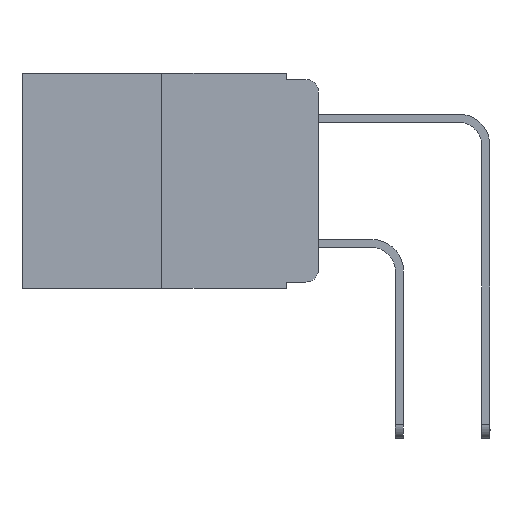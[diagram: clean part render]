
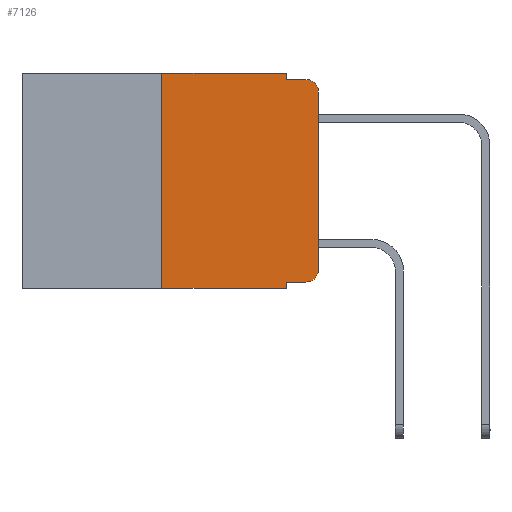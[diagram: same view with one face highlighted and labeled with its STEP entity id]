
A CAD part, left-side view. The second image highlights one B-rep face of the part: STEP entity #7126.
In plain terms, the highlighted planar face has unit normal (-1, 0, 0).
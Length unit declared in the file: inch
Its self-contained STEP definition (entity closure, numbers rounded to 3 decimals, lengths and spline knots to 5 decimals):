
#62 = ORIENTED_EDGE ( 'NONE', *, *, #11302, .T. ) ;
#249 = CARTESIAN_POINT ( 'NONE',  ( 0., 0.051, -0.01 ) ) ;
#327 = PLANE ( 'NONE',  #916 ) ;
#438 = AXIS2_PLACEMENT_3D ( 'NONE', #8226, #11312, #13132 ) ;
#916 = AXIS2_PLACEMENT_3D ( 'NONE', #1693, #9468, #11037 ) ;
#928 = DIRECTION ( 'NONE',  ( 0., 0., -1. ) ) ;
#1140 = LINE ( 'NONE', #249, #10842 ) ;
#1475 = CIRCLE ( 'NONE', #12382, 0.02 ) ;
#1693 = CARTESIAN_POINT ( 'NONE',  ( 0., 0.473, 0. ) ) ;
#1869 = EDGE_CURVE ( 'NONE', #2142, #2670, #3635, .T. ) ;
#2142 = VERTEX_POINT ( 'NONE', #12959 ) ;
#2294 = ORIENTED_EDGE ( 'NONE', *, *, #1869, .F. ) ;
#2642 = ORIENTED_EDGE ( 'NONE', *, *, #11221, .T. ) ;
#2658 = ORIENTED_EDGE ( 'NONE', *, *, #2874, .F. ) ;
#2670 = VERTEX_POINT ( 'NONE', #5640 ) ;
#2736 = VERTEX_POINT ( 'NONE', #5255 ) ;
#2874 = EDGE_CURVE ( 'NONE', #3925, #13097, #16921, .T. ) ;
#3635 = LINE ( 'NONE', #16708, #6300 ) ;
#3925 = VERTEX_POINT ( 'NONE', #10265 ) ;
#3939 = ORIENTED_EDGE ( 'NONE', *, *, #9696, .T. ) ;
#4692 = VERTEX_POINT ( 'NONE', #11938 ) ;
#4830 = CARTESIAN_POINT ( 'NONE',  ( 0., 0.25, -0.343 ) ) ;
#5009 = CARTESIAN_POINT ( 'NONE',  ( 0., 0.25, 0. ) ) ;
#5255 = CARTESIAN_POINT ( 'NONE',  ( 0., 0.02, -0.333 ) ) ;
#5284 = CARTESIAN_POINT ( 'NONE',  ( 0., 0.473, -0.343 ) ) ;
#5640 = CARTESIAN_POINT ( 'NONE',  ( 0., 0.051, -0.01 ) ) ;
#5737 = DIRECTION ( 'NONE',  ( 0., 0., -1. ) ) ;
#5816 = EDGE_CURVE ( 'NONE', #4692, #2142, #19254, .T. ) ;
#5990 = VECTOR ( 'NONE', #17746, 39.37008 ) ;
#6300 = VECTOR ( 'NONE', #19614, 39.37008 ) ;
#6592 = ORIENTED_EDGE ( 'NONE', *, *, #7976, .F. ) ;
#7126 = ADVANCED_FACE ( 'NONE', ( #15582 ), #327, .F. ) ;
#7976 = EDGE_CURVE ( 'NONE', #19413, #4692, #19197, .T. ) ;
#8202 = CARTESIAN_POINT ( 'NONE',  ( 0., 0., -0.313 ) ) ;
#8226 = CARTESIAN_POINT ( 'NONE',  ( 0., 0.02, -0.03 ) ) ;
#8430 = DIRECTION ( 'NONE',  ( -1., 0., 0. ) ) ;
#8497 = ORIENTED_EDGE ( 'NONE', *, *, #8825, .T. ) ;
#8541 = CARTESIAN_POINT ( 'NONE',  ( 0., 0.051, -0.333 ) ) ;
#8825 = EDGE_CURVE ( 'NONE', #2736, #11084, #1475, .T. ) ;
#9330 = EDGE_LOOP ( 'NONE', ( #16702, #3939, #11700, #2294, #16888, #6592, #62, #2658, #2642, #8497 ) ) ;
#9412 = VECTOR ( 'NONE', #5737, 39.37008 ) ;
#9468 = DIRECTION ( 'NONE',  ( 1., 0., 0. ) ) ;
#9590 = LINE ( 'NONE', #14490, #16376 ) ;
#9653 = DIRECTION ( 'NONE',  ( 0., -1., 0. ) ) ;
#9696 = EDGE_CURVE ( 'NONE', #13938, #11615, #12123, .T. ) ;
#9826 = DIRECTION ( 'NONE',  ( 0., -1., 0. ) ) ;
#10048 = VECTOR ( 'NONE', #10253, 39.37008 ) ;
#10253 = DIRECTION ( 'NONE',  ( 0., -1., 0. ) ) ;
#10265 = CARTESIAN_POINT ( 'NONE',  ( 0., 0.051, -0.333 ) ) ;
#10842 = VECTOR ( 'NONE', #9653, 39.37008 ) ;
#11037 = DIRECTION ( 'NONE',  ( 0., 0., -1. ) ) ;
#11084 = VERTEX_POINT ( 'NONE', #8202 ) ;
#11221 = EDGE_CURVE ( 'NONE', #3925, #2736, #18585, .T. ) ;
#11302 = EDGE_CURVE ( 'NONE', #19413, #13097, #16900, .T. ) ;
#11312 = DIRECTION ( 'NONE',  ( -1., 0., 0. ) ) ;
#11615 = VERTEX_POINT ( 'NONE', #16879 ) ;
#11700 = ORIENTED_EDGE ( 'NONE', *, *, #15990, .F. ) ;
#11822 = EDGE_CURVE ( 'NONE', #11084, #13938, #9590, .T. ) ;
#11938 = CARTESIAN_POINT ( 'NONE',  ( 0., 0.25, 0. ) ) ;
#12123 = CIRCLE ( 'NONE', #438, 0.02 ) ;
#12187 = CARTESIAN_POINT ( 'NONE',  ( 0., 0., -0.03 ) ) ;
#12382 = AXIS2_PLACEMENT_3D ( 'NONE', #19330, #8430, #928 ) ;
#12615 = DIRECTION ( 'NONE',  ( 0., 0., 1. ) ) ;
#12959 = CARTESIAN_POINT ( 'NONE',  ( 0., 0.051, 0. ) ) ;
#13097 = VERTEX_POINT ( 'NONE', #17825 ) ;
#13132 = DIRECTION ( 'NONE',  ( 0., 0., -1. ) ) ;
#13938 = VERTEX_POINT ( 'NONE', #12187 ) ;
#14490 = CARTESIAN_POINT ( 'NONE',  ( 0., 0., 0. ) ) ;
#15582 = FACE_OUTER_BOUND ( 'NONE', #9330, .T. ) ;
#15584 = VECTOR ( 'NONE', #12615, 39.37008 ) ;
#15990 = EDGE_CURVE ( 'NONE', #2670, #11615, #1140, .T. ) ;
#16042 = DIRECTION ( 'NONE',  ( 0., 0., 1. ) ) ;
#16376 = VECTOR ( 'NONE', #16042, 39.37008 ) ;
#16410 = VECTOR ( 'NONE', #9826, 39.37008 ) ;
#16445 = CARTESIAN_POINT ( 'NONE',  ( 0., 0.051, 0. ) ) ;
#16702 = ORIENTED_EDGE ( 'NONE', *, *, #11822, .T. ) ;
#16708 = CARTESIAN_POINT ( 'NONE',  ( 0., 0.051, 0. ) ) ;
#16879 = CARTESIAN_POINT ( 'NONE',  ( 0., 0.02, -0.01 ) ) ;
#16888 = ORIENTED_EDGE ( 'NONE', *, *, #5816, .F. ) ;
#16900 = LINE ( 'NONE', #5284, #16410 ) ;
#16921 = LINE ( 'NONE', #16445, #9412 ) ;
#17746 = DIRECTION ( 'NONE',  ( 0., -1., 0. ) ) ;
#17825 = CARTESIAN_POINT ( 'NONE',  ( 0., 0.051, -0.343 ) ) ;
#18039 = CARTESIAN_POINT ( 'NONE',  ( 0., 0.473, 0. ) ) ;
#18585 = LINE ( 'NONE', #8541, #5990 ) ;
#19197 = LINE ( 'NONE', #5009, #15584 ) ;
#19254 = LINE ( 'NONE', #18039, #10048 ) ;
#19330 = CARTESIAN_POINT ( 'NONE',  ( 0., 0.02, -0.313 ) ) ;
#19413 = VERTEX_POINT ( 'NONE', #4830 ) ;
#19614 = DIRECTION ( 'NONE',  ( 0., 0., -1. ) ) ;
